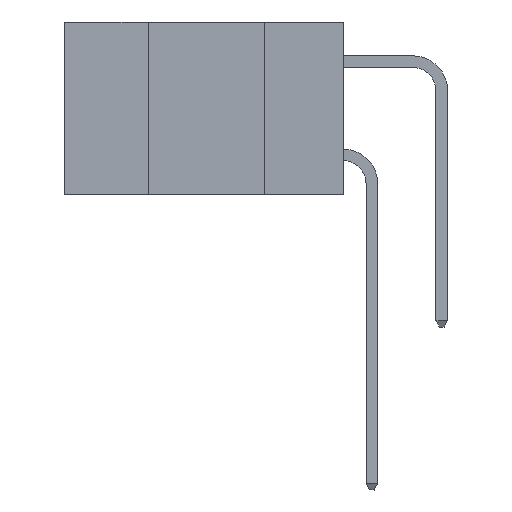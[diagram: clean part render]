
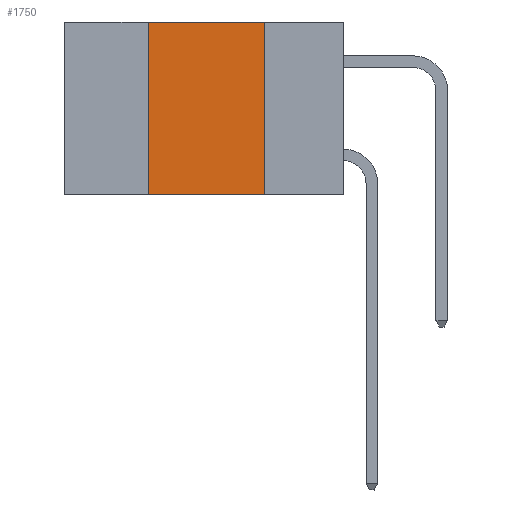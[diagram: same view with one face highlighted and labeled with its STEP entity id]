
A CAD part, left-side view. The second image highlights one B-rep face of the part: STEP entity #1750.
In plain terms, the highlighted planar face has unit normal (-1, 0, 0).
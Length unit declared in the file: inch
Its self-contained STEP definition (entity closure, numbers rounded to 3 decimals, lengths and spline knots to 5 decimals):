
#25 = DIRECTION ( 'NONE',  ( 0., 0., -1. ) ) ;
#172 = LINE ( 'NONE', #2712, #4445 ) ;
#1046 = VECTOR ( 'NONE', #7051, 39.37008 ) ;
#1397 = CARTESIAN_POINT ( 'NONE',  ( 0., 0.6, 0. ) ) ;
#1750 = ADVANCED_FACE ( 'NONE', ( #3094 ), #2394, .F. ) ;
#2048 = DIRECTION ( 'NONE',  ( 0., 0., 1. ) ) ;
#2170 = DIRECTION ( 'NONE',  ( 1., 0., 0. ) ) ;
#2394 = PLANE ( 'NONE',  #8986 ) ;
#2712 = CARTESIAN_POINT ( 'NONE',  ( 0., 0.6, -0.37 ) ) ;
#2953 = CARTESIAN_POINT ( 'NONE',  ( 0., 0.17, 0. ) ) ;
#3094 = FACE_OUTER_BOUND ( 'NONE', #8109, .T. ) ;
#3190 = CARTESIAN_POINT ( 'NONE',  ( 0., 0.42, -0.37 ) ) ;
#3586 = EDGE_CURVE ( 'NONE', #10110, #4311, #10241, .T. ) ;
#3862 = VECTOR ( 'NONE', #25, 39.37008 ) ;
#4078 = CARTESIAN_POINT ( 'NONE',  ( 0., 0.42, 0. ) ) ;
#4211 = ORIENTED_EDGE ( 'NONE', *, *, #8695, .T. ) ;
#4215 = CARTESIAN_POINT ( 'NONE',  ( 0., 0.6, 0. ) ) ;
#4311 = VERTEX_POINT ( 'NONE', #2953 ) ;
#4439 = LINE ( 'NONE', #7986, #3862 ) ;
#4445 = VECTOR ( 'NONE', #7902, 39.37008 ) ;
#5124 = ORIENTED_EDGE ( 'NONE', *, *, #3586, .F. ) ;
#5268 = VERTEX_POINT ( 'NONE', #6733 ) ;
#5656 = LINE ( 'NONE', #3190, #9435 ) ;
#6341 = CARTESIAN_POINT ( 'NONE',  ( 0., 0.42, -0.37 ) ) ;
#6455 = EDGE_CURVE ( 'NONE', #4311, #5268, #4439, .T. ) ;
#6733 = CARTESIAN_POINT ( 'NONE',  ( 0., 0.17, -0.37 ) ) ;
#6828 = VERTEX_POINT ( 'NONE', #6341 ) ;
#7051 = DIRECTION ( 'NONE',  ( 0., -1., 0. ) ) ;
#7796 = EDGE_CURVE ( 'NONE', #6828, #10110, #5656, .T. ) ;
#7902 = DIRECTION ( 'NONE',  ( 0., -1., 0. ) ) ;
#7986 = CARTESIAN_POINT ( 'NONE',  ( 0., 0.17, -0.37 ) ) ;
#8109 = EDGE_LOOP ( 'NONE', ( #10297, #5124, #9638, #4211 ) ) ;
#8695 = EDGE_CURVE ( 'NONE', #6828, #5268, #172, .T. ) ;
#8986 = AXIS2_PLACEMENT_3D ( 'NONE', #4215, #2170, #9314 ) ;
#9314 = DIRECTION ( 'NONE',  ( 0., 0., -1. ) ) ;
#9435 = VECTOR ( 'NONE', #2048, 39.37008 ) ;
#9638 = ORIENTED_EDGE ( 'NONE', *, *, #7796, .F. ) ;
#10110 = VERTEX_POINT ( 'NONE', #4078 ) ;
#10241 = LINE ( 'NONE', #1397, #1046 ) ;
#10297 = ORIENTED_EDGE ( 'NONE', *, *, #6455, .F. ) ;
